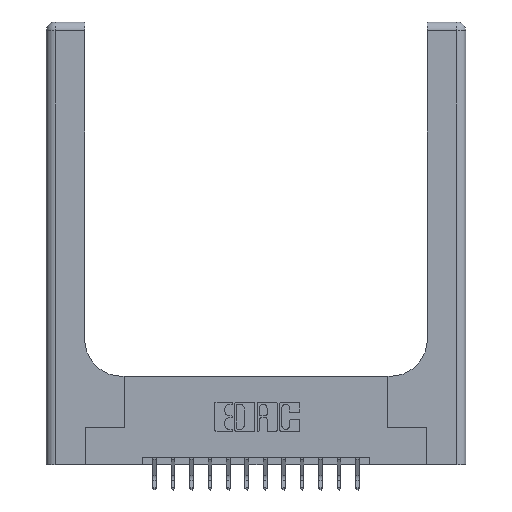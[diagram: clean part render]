
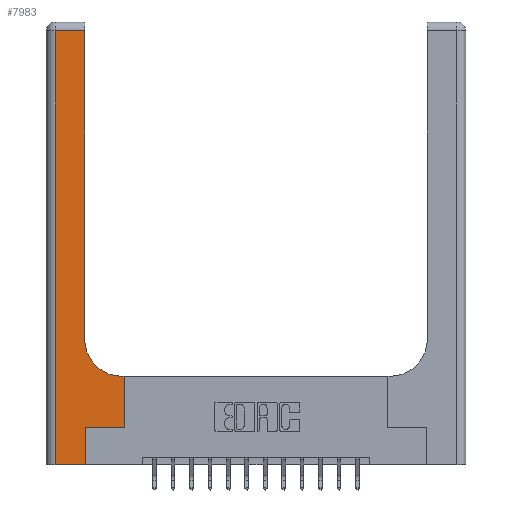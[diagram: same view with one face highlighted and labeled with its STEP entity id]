
A CAD part, top view. The second image highlights one B-rep face of the part: STEP entity #7983.
In plain terms, the highlighted planar face has unit normal (0, 0, 1).
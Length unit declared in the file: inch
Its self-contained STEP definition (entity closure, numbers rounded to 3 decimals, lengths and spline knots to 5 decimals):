
#539 = DIRECTION ( 'NONE',  ( 0., 0., -1. ) ) ;
#722 = CARTESIAN_POINT ( 'NONE',  ( 0.265, 0.25, 0.37 ) ) ;
#730 = CARTESIAN_POINT ( 'NONE',  ( 0., 2.94, 0.37 ) ) ;
#1307 = VECTOR ( 'NONE', #5018, 39.37008 ) ;
#1353 = CARTESIAN_POINT ( 'NONE',  ( 0.51, 0.6, 0.37 ) ) ;
#1848 = CARTESIAN_POINT ( 'NONE',  ( 0., 3., 0.37 ) ) ;
#1991 = LINE ( 'NONE', #730, #6270 ) ;
#2012 = VERTEX_POINT ( 'NONE', #722 ) ;
#2024 = CARTESIAN_POINT ( 'NONE',  ( 0.26, 2.94, 0.37 ) ) ;
#2424 = EDGE_CURVE ( 'NONE', #3149, #14220, #7166, .T. ) ;
#2776 = LINE ( 'NONE', #13627, #6359 ) ;
#3149 = VERTEX_POINT ( 'NONE', #4931 ) ;
#3448 = AXIS2_PLACEMENT_3D ( 'NONE', #13900, #539, #4571 ) ;
#3641 = VERTEX_POINT ( 'NONE', #17125 ) ;
#3691 = EDGE_CURVE ( 'NONE', #3641, #11784, #15687, .T. ) ;
#3988 = ORIENTED_EDGE ( 'NONE', *, *, #2424, .T. ) ;
#4401 = LINE ( 'NONE', #6911, #5074 ) ;
#4526 = VECTOR ( 'NONE', #11289, 39.37008 ) ;
#4571 = DIRECTION ( 'NONE',  ( 1., 0., 0. ) ) ;
#4869 = CIRCLE ( 'NONE', #3448, 0.25 ) ;
#4931 = CARTESIAN_POINT ( 'NONE',  ( 0.06, 2.94, 0.37 ) ) ;
#5018 = DIRECTION ( 'NONE',  ( 1., 0., 0. ) ) ;
#5074 = VECTOR ( 'NONE', #6999, 39.37008 ) ;
#5330 = EDGE_CURVE ( 'NONE', #17692, #3149, #1991, .T. ) ;
#5681 = CARTESIAN_POINT ( 'NONE',  ( 0.528, 0.6, 0.37 ) ) ;
#5792 = ORIENTED_EDGE ( 'NONE', *, *, #5330, .T. ) ;
#5969 = ORIENTED_EDGE ( 'NONE', *, *, #9046, .T. ) ;
#6012 = EDGE_CURVE ( 'NONE', #2012, #3641, #11005, .T. ) ;
#6095 = LINE ( 'NONE', #15239, #8408 ) ;
#6270 = VECTOR ( 'NONE', #15623, 39.37008 ) ;
#6359 = VECTOR ( 'NONE', #16410, 39.37008 ) ;
#6853 = EDGE_CURVE ( 'NONE', #14976, #17296, #4869, .T. ) ;
#6911 = CARTESIAN_POINT ( 'NONE',  ( 0.26, 0.6, 0.37 ) ) ;
#6999 = DIRECTION ( 'NONE',  ( -1., 0., 0. ) ) ;
#7166 = LINE ( 'NONE', #10127, #4526 ) ;
#7310 = DIRECTION ( 'NONE',  ( 0., 0., -1. ) ) ;
#7614 = CARTESIAN_POINT ( 'NONE',  ( 0.528, 0.25, 0.37 ) ) ;
#7983 = ADVANCED_FACE ( 'NONE', ( #15738 ), #14297, .F. ) ;
#8408 = VECTOR ( 'NONE', #14066, 39.37008 ) ;
#9046 = EDGE_CURVE ( 'NONE', #11784, #14976, #4401, .T. ) ;
#9384 = ORIENTED_EDGE ( 'NONE', *, *, #10262, .T. ) ;
#9558 = ORIENTED_EDGE ( 'NONE', *, *, #6853, .T. ) ;
#9630 = VECTOR ( 'NONE', #12721, 39.37008 ) ;
#10127 = CARTESIAN_POINT ( 'NONE',  ( 0.06, 3., 0.37 ) ) ;
#10262 = EDGE_CURVE ( 'NONE', #14220, #16056, #16899, .T. ) ;
#10351 = ORIENTED_EDGE ( 'NONE', *, *, #17159, .T. ) ;
#11005 = LINE ( 'NONE', #16839, #11452 ) ;
#11289 = DIRECTION ( 'NONE',  ( 0., -1., 0. ) ) ;
#11429 = DIRECTION ( 'NONE',  ( -1., 0., 0. ) ) ;
#11452 = VECTOR ( 'NONE', #15312, 39.37008 ) ;
#11784 = VERTEX_POINT ( 'NONE', #5681 ) ;
#12721 = DIRECTION ( 'NONE',  ( 0., 1., 0. ) ) ;
#12978 = CARTESIAN_POINT ( 'NONE',  ( 0.26, 0.85, 0.37 ) ) ;
#13174 = CARTESIAN_POINT ( 'NONE',  ( 0., 0., 0.37 ) ) ;
#13627 = CARTESIAN_POINT ( 'NONE',  ( 0.26, 3., 0.37 ) ) ;
#13900 = CARTESIAN_POINT ( 'NONE',  ( 0.51, 0.85, 0.37 ) ) ;
#14066 = DIRECTION ( 'NONE',  ( 0., 1., 0. ) ) ;
#14195 = AXIS2_PLACEMENT_3D ( 'NONE', #1848, #7310, #11429 ) ;
#14220 = VERTEX_POINT ( 'NONE', #16031 ) ;
#14297 = PLANE ( 'NONE',  #14195 ) ;
#14508 = ORIENTED_EDGE ( 'NONE', *, *, #3691, .T. ) ;
#14911 = CARTESIAN_POINT ( 'NONE',  ( 0.265, 0., 0.37 ) ) ;
#14947 = EDGE_CURVE ( 'NONE', #17296, #17692, #2776, .T. ) ;
#14976 = VERTEX_POINT ( 'NONE', #1353 ) ;
#15239 = CARTESIAN_POINT ( 'NONE',  ( 0.265, 0., 0.37 ) ) ;
#15312 = DIRECTION ( 'NONE',  ( 1., 0., 0. ) ) ;
#15623 = DIRECTION ( 'NONE',  ( -1., 0., 0. ) ) ;
#15687 = LINE ( 'NONE', #7614, #9630 ) ;
#15738 = FACE_OUTER_BOUND ( 'NONE', #16498, .T. ) ;
#16031 = CARTESIAN_POINT ( 'NONE',  ( 0.06, 0., 0.37 ) ) ;
#16056 = VERTEX_POINT ( 'NONE', #14911 ) ;
#16320 = ORIENTED_EDGE ( 'NONE', *, *, #14947, .T. ) ;
#16410 = DIRECTION ( 'NONE',  ( 0., 1., 0. ) ) ;
#16498 = EDGE_LOOP ( 'NONE', ( #16320, #5792, #3988, #9384, #10351, #17338, #14508, #5969, #9558 ) ) ;
#16839 = CARTESIAN_POINT ( 'NONE',  ( 0.265, 0.25, 0.37 ) ) ;
#16899 = LINE ( 'NONE', #13174, #1307 ) ;
#17125 = CARTESIAN_POINT ( 'NONE',  ( 0.528, 0.25, 0.37 ) ) ;
#17159 = EDGE_CURVE ( 'NONE', #16056, #2012, #6095, .T. ) ;
#17296 = VERTEX_POINT ( 'NONE', #12978 ) ;
#17338 = ORIENTED_EDGE ( 'NONE', *, *, #6012, .T. ) ;
#17692 = VERTEX_POINT ( 'NONE', #2024 ) ;
